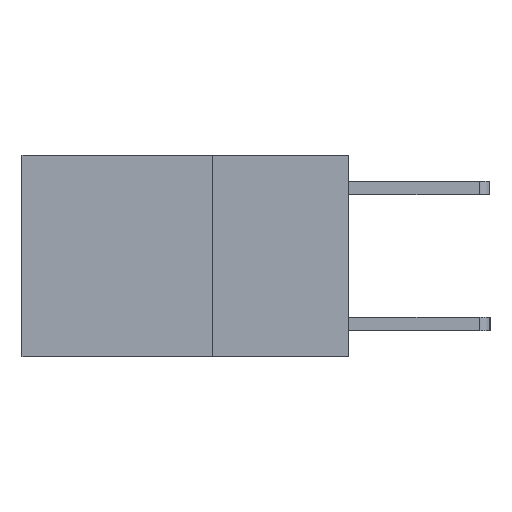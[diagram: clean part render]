
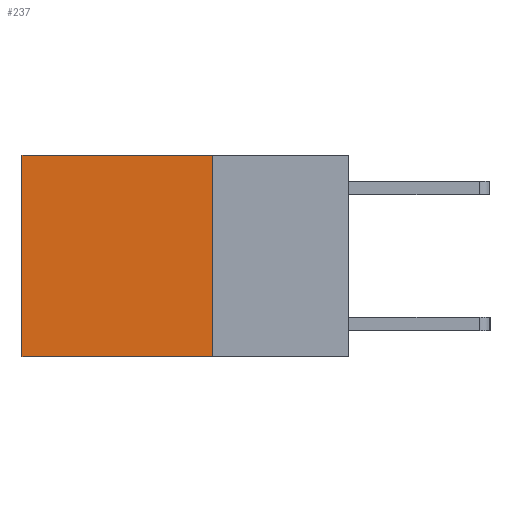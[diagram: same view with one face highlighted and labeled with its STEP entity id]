
A CAD part, left-side view. The second image highlights one B-rep face of the part: STEP entity #237.
In plain terms, the highlighted planar face has unit normal (-1, 0, 0).
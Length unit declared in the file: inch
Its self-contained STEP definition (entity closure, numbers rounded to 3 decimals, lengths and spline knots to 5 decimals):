
#30 = LINE ( 'NONE', #8312, #3465 ) ;
#146 = VERTEX_POINT ( 'NONE', #8332 ) ;
#237 = ADVANCED_FACE ( 'NONE', ( #769 ), #6490, .F. ) ;
#466 = EDGE_LOOP ( 'NONE', ( #5095, #6855, #605, #1944 ) ) ;
#605 = ORIENTED_EDGE ( 'NONE', *, *, #8001, .F. ) ;
#751 = LINE ( 'NONE', #7704, #2994 ) ;
#769 = FACE_OUTER_BOUND ( 'NONE', #466, .T. ) ;
#806 = VERTEX_POINT ( 'NONE', #3315 ) ;
#1570 = EDGE_CURVE ( 'NONE', #6942, #806, #751, .T. ) ;
#1944 = ORIENTED_EDGE ( 'NONE', *, *, #3896, .T. ) ;
#2614 = DIRECTION ( 'NONE',  ( 0., 1., 0. ) ) ;
#2784 = DIRECTION ( 'NONE',  ( 1., 0., 0. ) ) ;
#2828 = CARTESIAN_POINT ( 'NONE',  ( 0.2625, 0.25, 0. ) ) ;
#2856 = LINE ( 'NONE', #4158, #7811 ) ;
#2994 = VECTOR ( 'NONE', #6448, 39.37008 ) ;
#3155 = DIRECTION ( 'NONE',  ( 0., 1., 0. ) ) ;
#3315 = CARTESIAN_POINT ( 'NONE',  ( 0.2625, 0.6, -0.37 ) ) ;
#3465 = VECTOR ( 'NONE', #3155, 39.37008 ) ;
#3689 = CARTESIAN_POINT ( 'NONE',  ( 0.2625, 0.6, 0. ) ) ;
#3783 = AXIS2_PLACEMENT_3D ( 'NONE', #2828, #2784, #4160 ) ;
#3896 = EDGE_CURVE ( 'NONE', #6877, #6942, #30, .T. ) ;
#3953 = CARTESIAN_POINT ( 'NONE',  ( 0.2625, 0.25, -0.37 ) ) ;
#4158 = CARTESIAN_POINT ( 'NONE',  ( 0.2625, 0.25, 0. ) ) ;
#4160 = DIRECTION ( 'NONE',  ( 0., 0., -1. ) ) ;
#5095 = ORIENTED_EDGE ( 'NONE', *, *, #1570, .T. ) ;
#5581 = CARTESIAN_POINT ( 'NONE',  ( 0.2625, 0.25, 0. ) ) ;
#5923 = LINE ( 'NONE', #3953, #7419 ) ;
#6448 = DIRECTION ( 'NONE',  ( 0., 0., -1. ) ) ;
#6490 = PLANE ( 'NONE',  #3783 ) ;
#6625 = EDGE_CURVE ( 'NONE', #146, #806, #5923, .T. ) ;
#6855 = ORIENTED_EDGE ( 'NONE', *, *, #6625, .F. ) ;
#6877 = VERTEX_POINT ( 'NONE', #5581 ) ;
#6942 = VERTEX_POINT ( 'NONE', #3689 ) ;
#7419 = VECTOR ( 'NONE', #2614, 39.37008 ) ;
#7704 = CARTESIAN_POINT ( 'NONE',  ( 0.2625, 0.6, 0. ) ) ;
#7811 = VECTOR ( 'NONE', #7993, 39.37008 ) ;
#7993 = DIRECTION ( 'NONE',  ( 0., 0., -1. ) ) ;
#8001 = EDGE_CURVE ( 'NONE', #6877, #146, #2856, .T. ) ;
#8312 = CARTESIAN_POINT ( 'NONE',  ( 0.2625, 0.25, 0. ) ) ;
#8332 = CARTESIAN_POINT ( 'NONE',  ( 0.2625, 0.25, -0.37 ) ) ;
